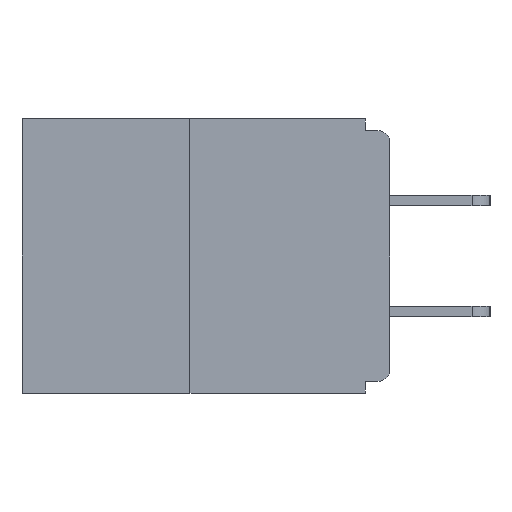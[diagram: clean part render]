
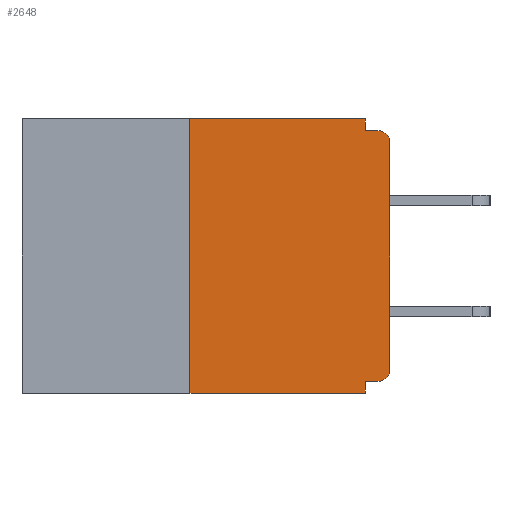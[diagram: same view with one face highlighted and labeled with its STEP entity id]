
A CAD part, left-side view. The second image highlights one B-rep face of the part: STEP entity #2648.
In plain terms, the highlighted planar face has unit normal (-1, 0, 0).
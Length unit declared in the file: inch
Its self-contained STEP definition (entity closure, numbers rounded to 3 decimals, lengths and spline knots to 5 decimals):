
#161 = CARTESIAN_POINT ( 'NONE',  ( 0., 0.46, -0.343 ) ) ;
#289 = ORIENTED_EDGE ( 'NONE', *, *, #10891, .F. ) ;
#535 = VERTEX_POINT ( 'NONE', #14142 ) ;
#657 = CARTESIAN_POINT ( 'NONE',  ( 0., 0.46, 0. ) ) ;
#875 = EDGE_CURVE ( 'NONE', #15035, #13220, #11071, .T. ) ;
#939 = DIRECTION ( 'NONE',  ( -1., 0., 0. ) ) ;
#1172 = LINE ( 'NONE', #12407, #19372 ) ;
#1716 = ORIENTED_EDGE ( 'NONE', *, *, #875, .T. ) ;
#2048 = VECTOR ( 'NONE', #11227, 39.37008 ) ;
#2244 = VERTEX_POINT ( 'NONE', #3137 ) ;
#2526 = ORIENTED_EDGE ( 'NONE', *, *, #17972, .T. ) ;
#2648 = ADVANCED_FACE ( 'NONE', ( #19412 ), #7269, .F. ) ;
#3137 = CARTESIAN_POINT ( 'NONE',  ( 0., 0.031, -0.328 ) ) ;
#3251 = CARTESIAN_POINT ( 'NONE',  ( 0., 0.031, 0. ) ) ;
#3309 = DIRECTION ( 'NONE',  ( 0., -1., 0. ) ) ;
#3856 = ORIENTED_EDGE ( 'NONE', *, *, #14865, .T. ) ;
#3979 = CARTESIAN_POINT ( 'NONE',  ( 0., 0.25, 0. ) ) ;
#4366 = DIRECTION ( 'NONE',  ( 0., 0., 1. ) ) ;
#4653 = DIRECTION ( 'NONE',  ( 0., 0., -1. ) ) ;
#4943 = EDGE_CURVE ( 'NONE', #535, #13534, #19318, .T. ) ;
#5013 = CARTESIAN_POINT ( 'NONE',  ( 0., 0., -0.313 ) ) ;
#5957 = VECTOR ( 'NONE', #13496, 39.37008 ) ;
#6427 = AXIS2_PLACEMENT_3D ( 'NONE', #10176, #939, #7163 ) ;
#7163 = DIRECTION ( 'NONE',  ( 0., 0., -1. ) ) ;
#7222 = VERTEX_POINT ( 'NONE', #8211 ) ;
#7269 = PLANE ( 'NONE',  #13276 ) ;
#7302 = VECTOR ( 'NONE', #3309, 39.37008 ) ;
#8211 = CARTESIAN_POINT ( 'NONE',  ( 0., 0.031, -0.343 ) ) ;
#8548 = VECTOR ( 'NONE', #18155, 39.37008 ) ;
#9065 = CARTESIAN_POINT ( 'NONE',  ( 0., 0.031, 0. ) ) ;
#9425 = ORIENTED_EDGE ( 'NONE', *, *, #14227, .F. ) ;
#9725 = VECTOR ( 'NONE', #12649, 39.37008 ) ;
#10061 = LINE ( 'NONE', #14980, #5957 ) ;
#10176 = CARTESIAN_POINT ( 'NONE',  ( 0., 0.015, -0.03 ) ) ;
#10478 = DIRECTION ( 'NONE',  ( 1., 0., 0. ) ) ;
#10638 = LINE ( 'NONE', #161, #7302 ) ;
#10683 = EDGE_CURVE ( 'NONE', #11180, #13534, #10061, .T. ) ;
#10696 = EDGE_CURVE ( 'NONE', #11058, #19141, #17223, .T. ) ;
#10891 = EDGE_CURVE ( 'NONE', #2244, #7222, #1172, .T. ) ;
#10942 = LINE ( 'NONE', #16336, #14976 ) ;
#11058 = VERTEX_POINT ( 'NONE', #19054 ) ;
#11071 = CIRCLE ( 'NONE', #16710, 0.015 ) ;
#11111 = ORIENTED_EDGE ( 'NONE', *, *, #10683, .F. ) ;
#11180 = VERTEX_POINT ( 'NONE', #17299 ) ;
#11227 = DIRECTION ( 'NONE',  ( 0., -1., 0. ) ) ;
#11723 = EDGE_CURVE ( 'NONE', #15035, #2244, #10942, .T. ) ;
#12289 = VERTEX_POINT ( 'NONE', #9065 ) ;
#12316 = LINE ( 'NONE', #657, #2048 ) ;
#12407 = CARTESIAN_POINT ( 'NONE',  ( 0., 0.031, -0.343 ) ) ;
#12649 = DIRECTION ( 'NONE',  ( 0., 0., 1. ) ) ;
#13067 = EDGE_CURVE ( 'NONE', #12289, #11180, #16658, .T. ) ;
#13220 = VERTEX_POINT ( 'NONE', #5013 ) ;
#13276 = AXIS2_PLACEMENT_3D ( 'NONE', #16538, #10478, #18078 ) ;
#13315 = DIRECTION ( 'NONE',  ( 0., 1., 0. ) ) ;
#13496 = DIRECTION ( 'NONE',  ( 0., -1., 0. ) ) ;
#13534 = VERTEX_POINT ( 'NONE', #18056 ) ;
#13718 = LINE ( 'NONE', #17231, #9725 ) ;
#13950 = CARTESIAN_POINT ( 'NONE',  ( 0., 0.015, -0.328 ) ) ;
#13982 = EDGE_LOOP ( 'NONE', ( #9425, #17184, #3856, #289, #15109, #1716, #2526, #16113, #11111, #17224 ) ) ;
#14142 = CARTESIAN_POINT ( 'NONE',  ( 0., 0., -0.03 ) ) ;
#14227 = EDGE_CURVE ( 'NONE', #19141, #12289, #12316, .T. ) ;
#14865 = EDGE_CURVE ( 'NONE', #11058, #7222, #10638, .T. ) ;
#14976 = VECTOR ( 'NONE', #13315, 39.37008 ) ;
#14980 = CARTESIAN_POINT ( 'NONE',  ( 0., 0., -0.015 ) ) ;
#15035 = VERTEX_POINT ( 'NONE', #13950 ) ;
#15109 = ORIENTED_EDGE ( 'NONE', *, *, #11723, .F. ) ;
#15387 = DIRECTION ( 'NONE',  ( 0., 0., -1. ) ) ;
#16113 = ORIENTED_EDGE ( 'NONE', *, *, #4943, .T. ) ;
#16336 = CARTESIAN_POINT ( 'NONE',  ( 0., 0., -0.328 ) ) ;
#16538 = CARTESIAN_POINT ( 'NONE',  ( 0., 0.46, 0. ) ) ;
#16590 = CARTESIAN_POINT ( 'NONE',  ( 0., 0.25, 0. ) ) ;
#16658 = LINE ( 'NONE', #3251, #8548 ) ;
#16710 = AXIS2_PLACEMENT_3D ( 'NONE', #18496, #18286, #15387 ) ;
#16718 = VECTOR ( 'NONE', #4366, 39.37008 ) ;
#17184 = ORIENTED_EDGE ( 'NONE', *, *, #10696, .F. ) ;
#17223 = LINE ( 'NONE', #16590, #16718 ) ;
#17224 = ORIENTED_EDGE ( 'NONE', *, *, #13067, .F. ) ;
#17231 = CARTESIAN_POINT ( 'NONE',  ( 0., 0., 0. ) ) ;
#17299 = CARTESIAN_POINT ( 'NONE',  ( 0., 0.031, -0.015 ) ) ;
#17972 = EDGE_CURVE ( 'NONE', #13220, #535, #13718, .T. ) ;
#18056 = CARTESIAN_POINT ( 'NONE',  ( 0., 0.015, -0.015 ) ) ;
#18078 = DIRECTION ( 'NONE',  ( 0., 0., -1. ) ) ;
#18155 = DIRECTION ( 'NONE',  ( 0., 0., -1. ) ) ;
#18286 = DIRECTION ( 'NONE',  ( -1., 0., 0. ) ) ;
#18496 = CARTESIAN_POINT ( 'NONE',  ( 0., 0.015, -0.313 ) ) ;
#19054 = CARTESIAN_POINT ( 'NONE',  ( 0., 0.25, -0.343 ) ) ;
#19141 = VERTEX_POINT ( 'NONE', #3979 ) ;
#19318 = CIRCLE ( 'NONE', #6427, 0.015 ) ;
#19372 = VECTOR ( 'NONE', #4653, 39.37008 ) ;
#19412 = FACE_OUTER_BOUND ( 'NONE', #13982, .T. ) ;
